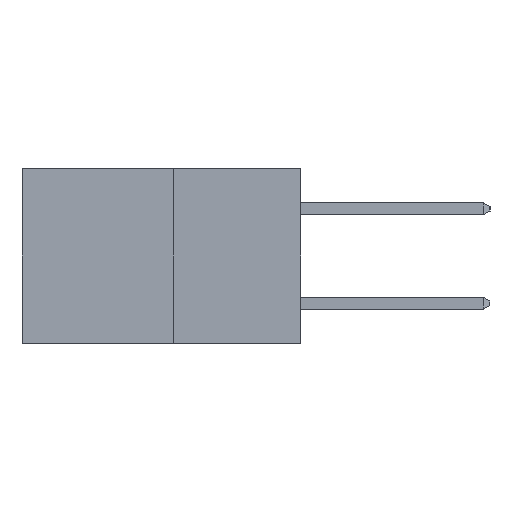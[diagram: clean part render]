
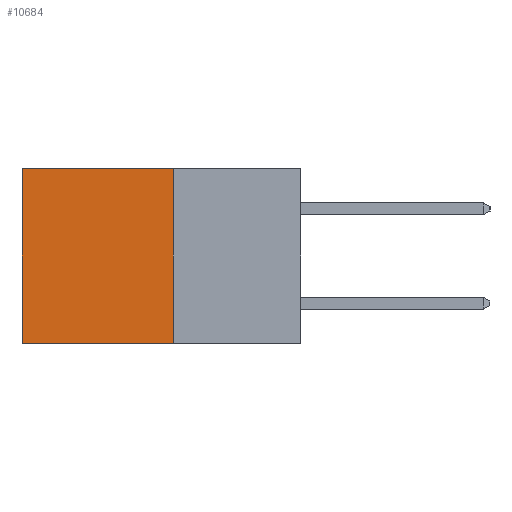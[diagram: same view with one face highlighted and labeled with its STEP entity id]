
A CAD part, left-side view. The second image highlights one B-rep face of the part: STEP entity #10684.
In plain terms, the highlighted planar face has unit normal (-1, 0, 0).
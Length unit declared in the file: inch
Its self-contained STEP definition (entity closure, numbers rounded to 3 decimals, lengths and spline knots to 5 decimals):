
#1069 = LINE ( 'NONE', #18431, #13025 ) ;
#1414 = VERTEX_POINT ( 'NONE', #18764 ) ;
#1590 = AXIS2_PLACEMENT_3D ( 'NONE', #18231, #9073, #19729 ) ;
#1830 = LINE ( 'NONE', #2207, #12302 ) ;
#2207 = CARTESIAN_POINT ( 'NONE',  ( 0.277, 0.59, -0.37 ) ) ;
#4060 = CARTESIAN_POINT ( 'NONE',  ( 0.277, 0.27, -0.37 ) ) ;
#5864 = ORIENTED_EDGE ( 'NONE', *, *, #16673, .T. ) ;
#6009 = VERTEX_POINT ( 'NONE', #18061 ) ;
#6181 = ORIENTED_EDGE ( 'NONE', *, *, #17648, .T. ) ;
#6457 = VECTOR ( 'NONE', #8770, 39.37008 ) ;
#6728 = CARTESIAN_POINT ( 'NONE',  ( 0.277, 0.59, 0. ) ) ;
#6966 = LINE ( 'NONE', #4060, #6457 ) ;
#7102 = VECTOR ( 'NONE', #10642, 39.37008 ) ;
#8594 = ORIENTED_EDGE ( 'NONE', *, *, #10070, .F. ) ;
#8770 = DIRECTION ( 'NONE',  ( 0., 1., 0. ) ) ;
#8843 = EDGE_LOOP ( 'NONE', ( #5864, #17694, #8594, #6181 ) ) ;
#9073 = DIRECTION ( 'NONE',  ( 1., 0., 0. ) ) ;
#9968 = DIRECTION ( 'NONE',  ( 0., 0., -1. ) ) ;
#10070 = EDGE_CURVE ( 'NONE', #10443, #1414, #1069, .T. ) ;
#10443 = VERTEX_POINT ( 'NONE', #19144 ) ;
#10578 = FACE_OUTER_BOUND ( 'NONE', #8843, .T. ) ;
#10642 = DIRECTION ( 'NONE',  ( 0., 1., 0. ) ) ;
#10684 = ADVANCED_FACE ( 'NONE', ( #10578 ), #18164, .F. ) ;
#11292 = LINE ( 'NONE', #12132, #7102 ) ;
#12132 = CARTESIAN_POINT ( 'NONE',  ( 0.277, 0.27, 0. ) ) ;
#12302 = VECTOR ( 'NONE', #9968, 39.37008 ) ;
#13025 = VECTOR ( 'NONE', #13929, 39.37008 ) ;
#13929 = DIRECTION ( 'NONE',  ( 0., 0., -1. ) ) ;
#15206 = EDGE_CURVE ( 'NONE', #1414, #6009, #6966, .T. ) ;
#16673 = EDGE_CURVE ( 'NONE', #18634, #6009, #1830, .T. ) ;
#17648 = EDGE_CURVE ( 'NONE', #10443, #18634, #11292, .T. ) ;
#17694 = ORIENTED_EDGE ( 'NONE', *, *, #15206, .F. ) ;
#18061 = CARTESIAN_POINT ( 'NONE',  ( 0.277, 0.59, -0.37 ) ) ;
#18164 = PLANE ( 'NONE',  #1590 ) ;
#18231 = CARTESIAN_POINT ( 'NONE',  ( 0.277, 0.27, -0.37 ) ) ;
#18431 = CARTESIAN_POINT ( 'NONE',  ( 0.277, 0.27, -0.37 ) ) ;
#18634 = VERTEX_POINT ( 'NONE', #6728 ) ;
#18764 = CARTESIAN_POINT ( 'NONE',  ( 0.277, 0.27, -0.37 ) ) ;
#19144 = CARTESIAN_POINT ( 'NONE',  ( 0.277, 0.27, 0. ) ) ;
#19729 = DIRECTION ( 'NONE',  ( 0., 0., -1. ) ) ;
